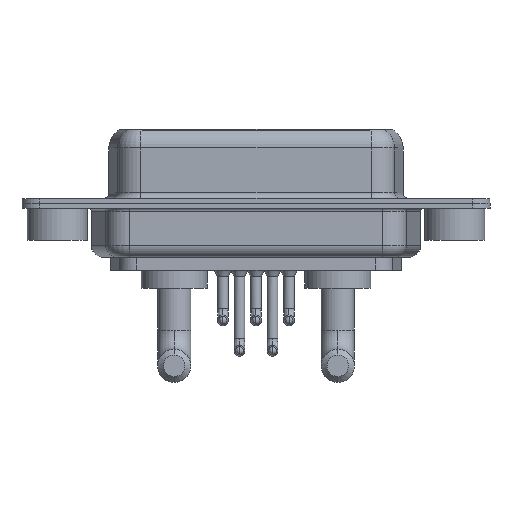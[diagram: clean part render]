
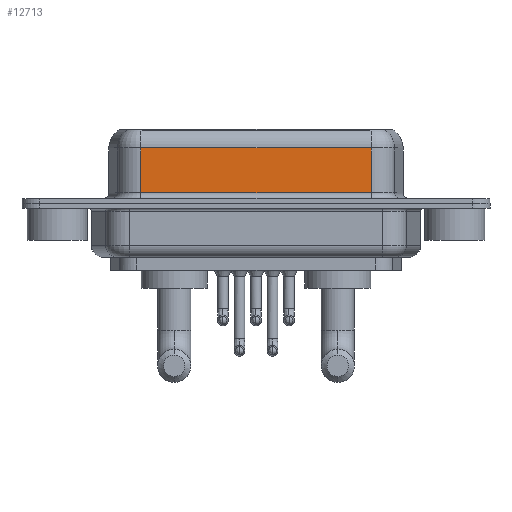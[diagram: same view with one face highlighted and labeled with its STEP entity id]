
A CAD part, front view. The second image highlights one B-rep face of the part: STEP entity #12713.
In plain terms, the highlighted planar face has unit normal (0, -1, 0).
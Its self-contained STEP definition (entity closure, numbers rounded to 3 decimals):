
#312 = EDGE_CURVE ( 'NONE', #6267, #13449, #4347, .T. ) ;
#365 = DIRECTION ( 'NONE',  ( 0., 0., -1. ) ) ;
#743 = CARTESIAN_POINT ( 'NONE',  ( 7.013, -3.95, 4.65 ) ) ;
#1422 = CARTESIAN_POINT ( 'NONE',  ( 26.287, -3.95, 0.9 ) ) ;
#1538 = EDGE_LOOP ( 'NONE', ( #5407, #5057, #13541, #14273 ) ) ;
#1786 = CARTESIAN_POINT ( 'NONE',  ( 26.287, -3.95, 4.65 ) ) ;
#1868 = CARTESIAN_POINT ( 'NONE',  ( 26.287, -3.95, 4.65 ) ) ;
#3522 = VECTOR ( 'NONE', #8663, 1000. ) ;
#4127 = CARTESIAN_POINT ( 'NONE',  ( 7.013, -3.95, 0.9 ) ) ;
#4287 = VECTOR ( 'NONE', #365, 1000. ) ;
#4347 = LINE ( 'NONE', #13512, #16535 ) ;
#5057 = ORIENTED_EDGE ( 'NONE', *, *, #13184, .T. ) ;
#5407 = ORIENTED_EDGE ( 'NONE', *, *, #7786, .F. ) ;
#5792 = DIRECTION ( 'NONE',  ( 1., 0., 0. ) ) ;
#6267 = VERTEX_POINT ( 'NONE', #4127 ) ;
#6806 = LINE ( 'NONE', #15810, #4287 ) ;
#6920 = DIRECTION ( 'NONE',  ( -1., 0., 0. ) ) ;
#7351 = DIRECTION ( 'NONE',  ( 0., 1., 0. ) ) ;
#7452 = VERTEX_POINT ( 'NONE', #743 ) ;
#7645 = CARTESIAN_POINT ( 'NONE',  ( 26.287, -3.95, 6.4 ) ) ;
#7786 = EDGE_CURVE ( 'NONE', #10774, #13449, #10135, .T. ) ;
#8663 = DIRECTION ( 'NONE',  ( 0., 0., -1. ) ) ;
#9736 = LINE ( 'NONE', #1868, #13291 ) ;
#10135 = LINE ( 'NONE', #7645, #3522 ) ;
#10774 = VERTEX_POINT ( 'NONE', #1786 ) ;
#11557 = CARTESIAN_POINT ( 'NONE',  ( 26.287, -3.95, 6.4 ) ) ;
#12665 = PLANE ( 'NONE',  #13012 ) ;
#12713 = ADVANCED_FACE ( 'NONE', ( #13861 ), #12665, .F. ) ;
#13012 = AXIS2_PLACEMENT_3D ( 'NONE', #11557, #7351, #16781 ) ;
#13184 = EDGE_CURVE ( 'NONE', #10774, #7452, #9736, .T. ) ;
#13291 = VECTOR ( 'NONE', #6920, 1000. ) ;
#13449 = VERTEX_POINT ( 'NONE', #1422 ) ;
#13512 = CARTESIAN_POINT ( 'NONE',  ( 26.287, -3.95, 0.9 ) ) ;
#13541 = ORIENTED_EDGE ( 'NONE', *, *, #14162, .T. ) ;
#13861 = FACE_OUTER_BOUND ( 'NONE', #1538, .T. ) ;
#14162 = EDGE_CURVE ( 'NONE', #7452, #6267, #6806, .T. ) ;
#14273 = ORIENTED_EDGE ( 'NONE', *, *, #312, .T. ) ;
#15810 = CARTESIAN_POINT ( 'NONE',  ( 7.013, -3.95, 6.4 ) ) ;
#16535 = VECTOR ( 'NONE', #5792, 1000. ) ;
#16781 = DIRECTION ( 'NONE',  ( 0., 0., 1. ) ) ;
